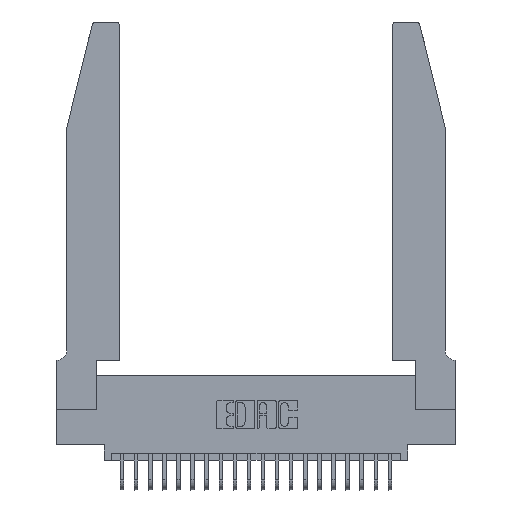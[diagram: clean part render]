
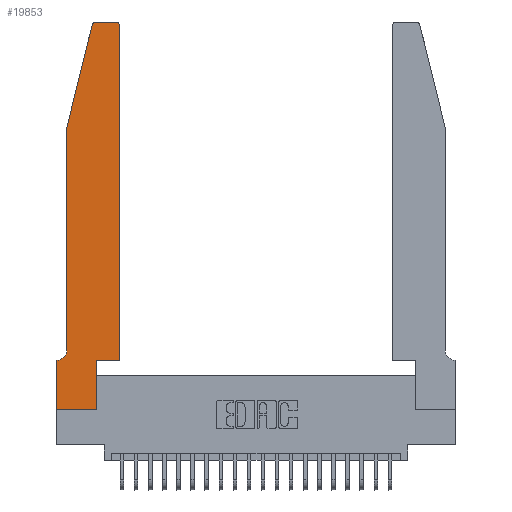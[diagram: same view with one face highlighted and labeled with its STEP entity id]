
A CAD part, top view. The second image highlights one B-rep face of the part: STEP entity #19853.
In plain terms, the highlighted planar face has unit normal (0, 0, 1).
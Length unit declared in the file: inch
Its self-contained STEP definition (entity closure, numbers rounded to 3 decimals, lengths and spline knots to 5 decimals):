
#145 = ORIENTED_EDGE ( 'NONE', *, *, #9370, .T. ) ;
#409 = CARTESIAN_POINT ( 'NONE',  ( 0.0755, 0.35, 0.37 ) ) ;
#439 = VECTOR ( 'NONE', #16223, 39.37008 ) ;
#570 = CARTESIAN_POINT ( 'NONE',  ( 0.284, 2.75, 0.37 ) ) ;
#839 = CIRCLE ( 'NONE', #1268, 0.07 ) ;
#896 = CIRCLE ( 'NONE', #9174, 0.03 ) ;
#1139 = CARTESIAN_POINT ( 'NONE',  ( 0.2865, 0.35, 0.37 ) ) ;
#1268 = AXIS2_PLACEMENT_3D ( 'NONE', #21908, #12427, #10579 ) ;
#1880 = CARTESIAN_POINT ( 'NONE',  ( 0., 0., 0.37 ) ) ;
#2040 = DIRECTION ( 'NONE',  ( 0., 0., 1. ) ) ;
#2218 = CARTESIAN_POINT ( 'NONE',  ( 0., 0.35, 0.37 ) ) ;
#2291 = ORIENTED_EDGE ( 'NONE', *, *, #22685, .T. ) ;
#2369 = LINE ( 'NONE', #14854, #22400 ) ;
#2628 = LINE ( 'NONE', #409, #439 ) ;
#2762 = DIRECTION ( 'NONE',  ( 0., -1., 0. ) ) ;
#2837 = VECTOR ( 'NONE', #12397, 39.37008 ) ;
#2889 = DIRECTION ( 'NONE',  ( 0., -1., 0. ) ) ;
#3213 = VERTEX_POINT ( 'NONE', #21804 ) ;
#3702 = EDGE_CURVE ( 'NONE', #11047, #8931, #21431, .T. ) ;
#4227 = CARTESIAN_POINT ( 'NONE',  ( 0.2605, 2.75, 0.37 ) ) ;
#4413 = VECTOR ( 'NONE', #12800, 39.37008 ) ;
#4622 = CARTESIAN_POINT ( 'NONE',  ( 0.284, 2.72, 0.37 ) ) ;
#5014 = LINE ( 'NONE', #16696, #4413 ) ;
#5505 = CIRCLE ( 'NONE', #12935, 0.03 ) ;
#5615 = ORIENTED_EDGE ( 'NONE', *, *, #13408, .T. ) ;
#6281 = VECTOR ( 'NONE', #2762, 39.37008 ) ;
#6400 = CARTESIAN_POINT ( 'NONE',  ( 0.2865, 0.35, 0.37 ) ) ;
#6623 = ORIENTED_EDGE ( 'NONE', *, *, #6892, .T. ) ;
#6892 = EDGE_CURVE ( 'NONE', #15604, #19684, #839, .T. ) ;
#7656 = VECTOR ( 'NONE', #23582, 39.37008 ) ;
#7691 = CARTESIAN_POINT ( 'NONE',  ( 0., 0., 0.37 ) ) ;
#7726 = EDGE_CURVE ( 'NONE', #12903, #11047, #2369, .T. ) ;
#7941 = EDGE_LOOP ( 'NONE', ( #14502, #5615, #12040, #19362, #6623, #20055, #145, #13438, #12992, #22831, #9058, #2291 ) ) ;
#8242 = LINE ( 'NONE', #4227, #7656 ) ;
#8579 = CARTESIAN_POINT ( 'NONE',  ( 0.0755, 2., 0.37 ) ) ;
#8931 = VERTEX_POINT ( 'NONE', #15786 ) ;
#8957 = FACE_OUTER_BOUND ( 'NONE', #7941, .T. ) ;
#9058 = ORIENTED_EDGE ( 'NONE', *, *, #3702, .T. ) ;
#9112 = CARTESIAN_POINT ( 'NONE',  ( 0.0055, 0.35, 0.37 ) ) ;
#9174 = AXIS2_PLACEMENT_3D ( 'NONE', #14465, #18382, #20335 ) ;
#9370 = EDGE_CURVE ( 'NONE', #22897, #15167, #12025, .T. ) ;
#9418 = CARTESIAN_POINT ( 'NONE',  ( 0.4505, 0.35, 0.37 ) ) ;
#9993 = CARTESIAN_POINT ( 'NONE',  ( 0.0755, 2., 0.37 ) ) ;
#10579 = DIRECTION ( 'NONE',  ( -1., 0., 0. ) ) ;
#10762 = CARTESIAN_POINT ( 'NONE',  ( 0.4505, 0.35, 0.37 ) ) ;
#10808 = EDGE_CURVE ( 'NONE', #23283, #12903, #16155, .T. ) ;
#11047 = VERTEX_POINT ( 'NONE', #10762 ) ;
#11115 = VECTOR ( 'NONE', #11389, 39.37008 ) ;
#11389 = DIRECTION ( 'NONE',  ( 0., 1., 0. ) ) ;
#11839 = DIRECTION ( 'NONE',  ( 0., 0., 1. ) ) ;
#12025 = LINE ( 'NONE', #22205, #19612 ) ;
#12040 = ORIENTED_EDGE ( 'NONE', *, *, #20256, .T. ) ;
#12397 = DIRECTION ( 'NONE',  ( 0., 1., 0. ) ) ;
#12427 = DIRECTION ( 'NONE',  ( 0., 0., -1. ) ) ;
#12800 = DIRECTION ( 'NONE',  ( -0.239, -0.971, 0. ) ) ;
#12903 = VERTEX_POINT ( 'NONE', #1139 ) ;
#12935 = AXIS2_PLACEMENT_3D ( 'NONE', #4622, #11839, #21491 ) ;
#12992 = ORIENTED_EDGE ( 'NONE', *, *, #10808, .T. ) ;
#13408 = EDGE_CURVE ( 'NONE', #13762, #3213, #5505, .T. ) ;
#13438 = ORIENTED_EDGE ( 'NONE', *, *, #22871, .T. ) ;
#13744 = EDGE_CURVE ( 'NONE', #13895, #13762, #8242, .T. ) ;
#13762 = VERTEX_POINT ( 'NONE', #570 ) ;
#13895 = VERTEX_POINT ( 'NONE', #21906 ) ;
#14274 = LINE ( 'NONE', #7691, #17933 ) ;
#14465 = CARTESIAN_POINT ( 'NONE',  ( 0.4205, 2.72, 0.37 ) ) ;
#14502 = ORIENTED_EDGE ( 'NONE', *, *, #13744, .T. ) ;
#14854 = CARTESIAN_POINT ( 'NONE',  ( 0.4505, 0.35, 0.37 ) ) ;
#15167 = VERTEX_POINT ( 'NONE', #1880 ) ;
#15604 = VERTEX_POINT ( 'NONE', #23741 ) ;
#15786 = CARTESIAN_POINT ( 'NONE',  ( 0.4505, 2.72, 0.37 ) ) ;
#16155 = LINE ( 'NONE', #6400, #2837 ) ;
#16223 = DIRECTION ( 'NONE',  ( -1., 0., 0. ) ) ;
#16398 = EDGE_CURVE ( 'NONE', #19684, #22897, #2628, .T. ) ;
#16548 = CARTESIAN_POINT ( 'NONE',  ( 0.2865, 0., 0.37 ) ) ;
#16696 = CARTESIAN_POINT ( 'NONE',  ( 0.0755, 2., 0.37 ) ) ;
#16811 = EDGE_CURVE ( 'NONE', #20148, #15604, #22008, .T. ) ;
#17933 = VECTOR ( 'NONE', #20903, 39.37008 ) ;
#18382 = DIRECTION ( 'NONE',  ( 0., 0., 1. ) ) ;
#19362 = ORIENTED_EDGE ( 'NONE', *, *, #16811, .T. ) ;
#19381 = PLANE ( 'NONE',  #22267 ) ;
#19612 = VECTOR ( 'NONE', #2889, 39.37008 ) ;
#19684 = VERTEX_POINT ( 'NONE', #9112 ) ;
#19853 = ADVANCED_FACE ( 'NONE', ( #8957 ), #19381, .T. ) ;
#20055 = ORIENTED_EDGE ( 'NONE', *, *, #16398, .T. ) ;
#20148 = VERTEX_POINT ( 'NONE', #8579 ) ;
#20256 = EDGE_CURVE ( 'NONE', #3213, #20148, #5014, .T. ) ;
#20335 = DIRECTION ( 'NONE',  ( 1., 0., 0. ) ) ;
#20903 = DIRECTION ( 'NONE',  ( 1., 0., 0. ) ) ;
#21161 = CARTESIAN_POINT ( 'NONE',  ( 0., 0.35, 0.37 ) ) ;
#21431 = LINE ( 'NONE', #9418, #11115 ) ;
#21491 = DIRECTION ( 'NONE',  ( 1., 0., 0. ) ) ;
#21804 = CARTESIAN_POINT ( 'NONE',  ( 0.25487, 2.72718, 0.37 ) ) ;
#21906 = CARTESIAN_POINT ( 'NONE',  ( 0.4205, 2.75, 0.37 ) ) ;
#21908 = CARTESIAN_POINT ( 'NONE',  ( 0.0055, 0.42, 0.37 ) ) ;
#22008 = LINE ( 'NONE', #9993, #6281 ) ;
#22205 = CARTESIAN_POINT ( 'NONE',  ( 0., 0., 0.37 ) ) ;
#22267 = AXIS2_PLACEMENT_3D ( 'NONE', #2218, #2040, #23289 ) ;
#22400 = VECTOR ( 'NONE', #24406, 39.37008 ) ;
#22685 = EDGE_CURVE ( 'NONE', #8931, #13895, #896, .T. ) ;
#22831 = ORIENTED_EDGE ( 'NONE', *, *, #7726, .T. ) ;
#22871 = EDGE_CURVE ( 'NONE', #15167, #23283, #14274, .T. ) ;
#22897 = VERTEX_POINT ( 'NONE', #21161 ) ;
#23283 = VERTEX_POINT ( 'NONE', #16548 ) ;
#23289 = DIRECTION ( 'NONE',  ( 1., 0., 0. ) ) ;
#23582 = DIRECTION ( 'NONE',  ( -1., 0., 0. ) ) ;
#23741 = CARTESIAN_POINT ( 'NONE',  ( 0.0755, 0.42, 0.37 ) ) ;
#24406 = DIRECTION ( 'NONE',  ( 1., 0., 0. ) ) ;
